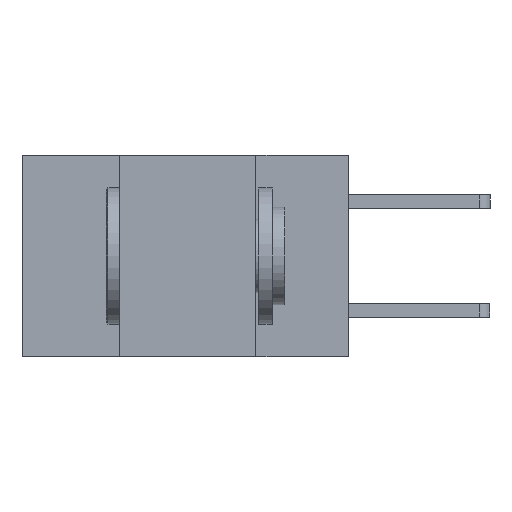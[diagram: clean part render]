
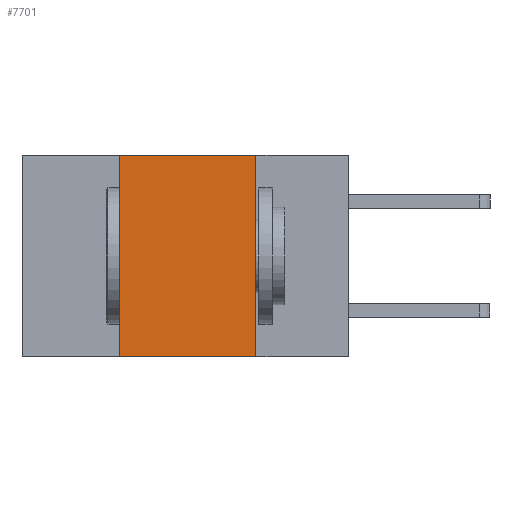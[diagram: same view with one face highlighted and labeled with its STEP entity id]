
A CAD part, left-side view. The second image highlights one B-rep face of the part: STEP entity #7701.
In plain terms, the highlighted planar face has unit normal (-1, 0, 0).
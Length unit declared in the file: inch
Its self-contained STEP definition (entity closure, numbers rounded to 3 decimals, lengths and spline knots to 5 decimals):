
#112 = DIRECTION ( 'NONE',  ( 0., 0., -1. ) ) ;
#132 = DIRECTION ( 'NONE',  ( 0., 0., -1. ) ) ;
#315 = EDGE_LOOP ( 'NONE', ( #729, #5158, #1022, #9180 ) ) ;
#729 = ORIENTED_EDGE ( 'NONE', *, *, #2752, .F. ) ;
#959 = CARTESIAN_POINT ( 'NONE',  ( 0., 0.6, 0. ) ) ;
#1022 = ORIENTED_EDGE ( 'NONE', *, *, #4071, .F. ) ;
#1535 = VECTOR ( 'NONE', #4920, 39.37008 ) ;
#1765 = CARTESIAN_POINT ( 'NONE',  ( 0., 0.17, 0. ) ) ;
#2704 = CARTESIAN_POINT ( 'NONE',  ( 0., 0.42, -0.37 ) ) ;
#2752 = EDGE_CURVE ( 'NONE', #5074, #2840, #6026, .T. ) ;
#2831 = CARTESIAN_POINT ( 'NONE',  ( 0., 0.17, -0.37 ) ) ;
#2840 = VERTEX_POINT ( 'NONE', #2831 ) ;
#3707 = FACE_OUTER_BOUND ( 'NONE', #315, .T. ) ;
#3751 = VECTOR ( 'NONE', #9769, 39.37008 ) ;
#4071 = EDGE_CURVE ( 'NONE', #6601, #7559, #7584, .T. ) ;
#4282 = CARTESIAN_POINT ( 'NONE',  ( 0., 0.6, 0. ) ) ;
#4878 = DIRECTION ( 'NONE',  ( 1., 0., 0. ) ) ;
#4920 = DIRECTION ( 'NONE',  ( 0., -1., 0. ) ) ;
#5074 = VERTEX_POINT ( 'NONE', #6387 ) ;
#5158 = ORIENTED_EDGE ( 'NONE', *, *, #6673, .F. ) ;
#6026 = LINE ( 'NONE', #1765, #9581 ) ;
#6387 = CARTESIAN_POINT ( 'NONE',  ( 0., 0.17, 0. ) ) ;
#6601 = VERTEX_POINT ( 'NONE', #2704 ) ;
#6673 = EDGE_CURVE ( 'NONE', #7559, #5074, #8949, .T. ) ;
#6939 = CARTESIAN_POINT ( 'NONE',  ( 0., 0.42, 0. ) ) ;
#7153 = PLANE ( 'NONE',  #8759 ) ;
#7559 = VERTEX_POINT ( 'NONE', #6939 ) ;
#7584 = LINE ( 'NONE', #9758, #3751 ) ;
#7701 = ADVANCED_FACE ( 'NONE', ( #3707 ), #7153, .F. ) ;
#8759 = AXIS2_PLACEMENT_3D ( 'NONE', #959, #4878, #112 ) ;
#8838 = DIRECTION ( 'NONE',  ( 0., -1., 0. ) ) ;
#8949 = LINE ( 'NONE', #4282, #9196 ) ;
#9038 = EDGE_CURVE ( 'NONE', #6601, #2840, #9843, .T. ) ;
#9180 = ORIENTED_EDGE ( 'NONE', *, *, #9038, .T. ) ;
#9196 = VECTOR ( 'NONE', #8838, 39.37008 ) ;
#9454 = CARTESIAN_POINT ( 'NONE',  ( 0., 0.6, -0.37 ) ) ;
#9581 = VECTOR ( 'NONE', #132, 39.37008 ) ;
#9758 = CARTESIAN_POINT ( 'NONE',  ( 0., 0.42, 0. ) ) ;
#9769 = DIRECTION ( 'NONE',  ( 0., 0., 1. ) ) ;
#9843 = LINE ( 'NONE', #9454, #1535 ) ;
